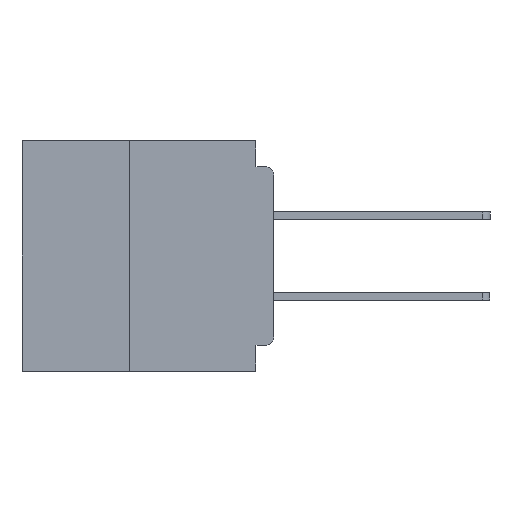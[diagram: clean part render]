
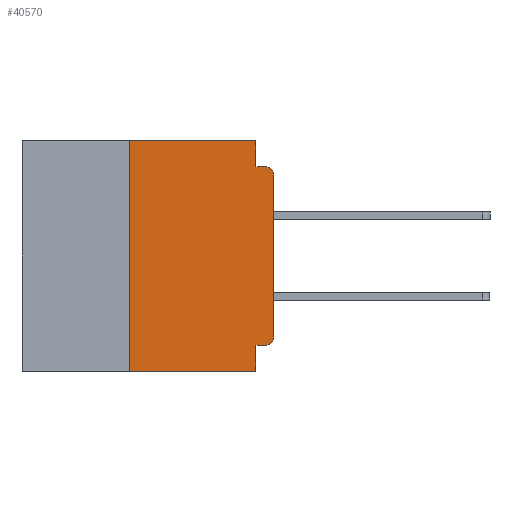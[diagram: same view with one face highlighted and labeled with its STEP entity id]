
A CAD part, left-side view. The second image highlights one B-rep face of the part: STEP entity #40570.
In plain terms, the highlighted planar face has unit normal (-1, 0, 0).
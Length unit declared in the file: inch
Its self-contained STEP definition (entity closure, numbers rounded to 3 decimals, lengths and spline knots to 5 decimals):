
#1601 = ORIENTED_EDGE ( 'NONE', *, *, #33294, .F. ) ;
#2261 = ORIENTED_EDGE ( 'NONE', *, *, #34584, .F. ) ;
#2350 = CARTESIAN_POINT ( 'NONE',  ( 0., 0.015, -0.355 ) ) ;
#2472 = EDGE_CURVE ( 'NONE', #12724, #2857, #5840, .T. ) ;
#2710 = VERTEX_POINT ( 'NONE', #24116 ) ;
#2857 = VERTEX_POINT ( 'NONE', #39718 ) ;
#2903 = AXIS2_PLACEMENT_3D ( 'NONE', #38630, #16112, #42362 ) ;
#3112 = VERTEX_POINT ( 'NONE', #37386 ) ;
#3600 = DIRECTION ( 'NONE',  ( 0., -1., 0. ) ) ;
#3895 = LINE ( 'NONE', #8994, #32750 ) ;
#4133 = ORIENTED_EDGE ( 'NONE', *, *, #35096, .F. ) ;
#4624 = VECTOR ( 'NONE', #18092, 39.37008 ) ;
#5840 = LINE ( 'NONE', #14567, #34676 ) ;
#6154 = DIRECTION ( 'NONE',  ( 1., 0., 0. ) ) ;
#6408 = CARTESIAN_POINT ( 'NONE',  ( 0., 0., -0.34 ) ) ;
#7140 = ORIENTED_EDGE ( 'NONE', *, *, #2472, .F. ) ;
#7187 = VECTOR ( 'NONE', #15323, 39.37008 ) ;
#8994 = CARTESIAN_POINT ( 'NONE',  ( 0., 0., -0.355 ) ) ;
#10626 = FACE_OUTER_BOUND ( 'NONE', #37354, .T. ) ;
#10797 = VERTEX_POINT ( 'NONE', #39583 ) ;
#11197 = VECTOR ( 'NONE', #3600, 39.37008 ) ;
#11697 = DIRECTION ( 'NONE',  ( -1., 0., 0. ) ) ;
#12574 = CARTESIAN_POINT ( 'NONE',  ( 0., 0.031, -0.4 ) ) ;
#12724 = VERTEX_POINT ( 'NONE', #30370 ) ;
#14567 = CARTESIAN_POINT ( 'NONE',  ( 0., 0.031, 0. ) ) ;
#14879 = CARTESIAN_POINT ( 'NONE',  ( 0., 0.437, 0. ) ) ;
#15323 = DIRECTION ( 'NONE',  ( 0., -1., 0. ) ) ;
#15664 = ORIENTED_EDGE ( 'NONE', *, *, #21819, .T. ) ;
#15750 = ORIENTED_EDGE ( 'NONE', *, *, #23505, .T. ) ;
#16112 = DIRECTION ( 'NONE',  ( -1., 0., 0. ) ) ;
#16523 = DIRECTION ( 'NONE',  ( 0., 1., 0. ) ) ;
#16916 = LINE ( 'NONE', #41896, #18067 ) ;
#17163 = LINE ( 'NONE', #30297, #7187 ) ;
#18067 = VECTOR ( 'NONE', #19364, 39.37008 ) ;
#18092 = DIRECTION ( 'NONE',  ( 0., 0., 1. ) ) ;
#18331 = DIRECTION ( 'NONE',  ( 0., 0., -1. ) ) ;
#18573 = CARTESIAN_POINT ( 'NONE',  ( 0., 0.437, -0.4 ) ) ;
#19364 = DIRECTION ( 'NONE',  ( 0., 0., 1. ) ) ;
#20019 = VERTEX_POINT ( 'NONE', #36186 ) ;
#21173 = LINE ( 'NONE', #18573, #11197 ) ;
#21819 = EDGE_CURVE ( 'NONE', #45614, #41257, #32991, .T. ) ;
#22986 = EDGE_CURVE ( 'NONE', #3112, #10797, #24855, .T. ) ;
#23505 = EDGE_CURVE ( 'NONE', #33548, #41833, #32451, .T. ) ;
#24116 = CARTESIAN_POINT ( 'NONE',  ( 0., 0.25, -0.4 ) ) ;
#24855 = LINE ( 'NONE', #12574, #33668 ) ;
#25273 = AXIS2_PLACEMENT_3D ( 'NONE', #28672, #6154, #32432 ) ;
#26003 = ORIENTED_EDGE ( 'NONE', *, *, #30054, .T. ) ;
#28672 = CARTESIAN_POINT ( 'NONE',  ( 0., 0.437, 0. ) ) ;
#30054 = EDGE_CURVE ( 'NONE', #41257, #33548, #16916, .T. ) ;
#30297 = CARTESIAN_POINT ( 'NONE',  ( 0., 0., -0.045 ) ) ;
#30370 = CARTESIAN_POINT ( 'NONE',  ( 0., 0.031, 0. ) ) ;
#32432 = DIRECTION ( 'NONE',  ( 0., 0., -1. ) ) ;
#32451 = CIRCLE ( 'NONE', #41072, 0.015 ) ;
#32750 = VECTOR ( 'NONE', #16523, 39.37008 ) ;
#32991 = CIRCLE ( 'NONE', #2903, 0.015 ) ;
#33294 = EDGE_CURVE ( 'NONE', #2857, #41833, #17163, .T. ) ;
#33454 = LINE ( 'NONE', #40608, #4624 ) ;
#33548 = VERTEX_POINT ( 'NONE', #35552 ) ;
#33668 = VECTOR ( 'NONE', #42586, 39.37008 ) ;
#34199 = CARTESIAN_POINT ( 'NONE',  ( 0., 0.015, -0.06 ) ) ;
#34584 = EDGE_CURVE ( 'NONE', #20019, #12724, #39385, .T. ) ;
#34676 = VECTOR ( 'NONE', #18331, 39.37008 ) ;
#35096 = EDGE_CURVE ( 'NONE', #2710, #20019, #33454, .T. ) ;
#35528 = ORIENTED_EDGE ( 'NONE', *, *, #22986, .F. ) ;
#35552 = CARTESIAN_POINT ( 'NONE',  ( 0., 0., -0.06 ) ) ;
#35618 = ORIENTED_EDGE ( 'NONE', *, *, #40800, .T. ) ;
#36166 = EDGE_CURVE ( 'NONE', #45614, #3112, #3895, .T. ) ;
#36186 = CARTESIAN_POINT ( 'NONE',  ( 0., 0.25, 0. ) ) ;
#37354 = EDGE_LOOP ( 'NONE', ( #26003, #15750, #1601, #7140, #2261, #4133, #35618, #35528, #38744, #15664 ) ) ;
#37386 = CARTESIAN_POINT ( 'NONE',  ( 0., 0.031, -0.355 ) ) ;
#37974 = DIRECTION ( 'NONE',  ( 0., 0., -1. ) ) ;
#38630 = CARTESIAN_POINT ( 'NONE',  ( 0., 0.015, -0.34 ) ) ;
#38744 = ORIENTED_EDGE ( 'NONE', *, *, #36166, .F. ) ;
#39385 = LINE ( 'NONE', #14879, #48148 ) ;
#39583 = CARTESIAN_POINT ( 'NONE',  ( 0., 0.031, -0.4 ) ) ;
#39718 = CARTESIAN_POINT ( 'NONE',  ( 0., 0.031, -0.045 ) ) ;
#39837 = PLANE ( 'NONE',  #25273 ) ;
#40570 = ADVANCED_FACE ( 'NONE', ( #10626 ), #39837, .F. ) ;
#40608 = CARTESIAN_POINT ( 'NONE',  ( 0., 0.25, -0.4 ) ) ;
#40800 = EDGE_CURVE ( 'NONE', #2710, #10797, #21173, .T. ) ;
#41072 = AXIS2_PLACEMENT_3D ( 'NONE', #34199, #11697, #37974 ) ;
#41143 = DIRECTION ( 'NONE',  ( 0., -1., 0. ) ) ;
#41257 = VERTEX_POINT ( 'NONE', #6408 ) ;
#41833 = VERTEX_POINT ( 'NONE', #47282 ) ;
#41896 = CARTESIAN_POINT ( 'NONE',  ( 0., 0., 0. ) ) ;
#42362 = DIRECTION ( 'NONE',  ( 0., 0., -1. ) ) ;
#42586 = DIRECTION ( 'NONE',  ( 0., 0., -1. ) ) ;
#45614 = VERTEX_POINT ( 'NONE', #2350 ) ;
#47282 = CARTESIAN_POINT ( 'NONE',  ( 0., 0.015, -0.045 ) ) ;
#48148 = VECTOR ( 'NONE', #41143, 39.37008 ) ;
